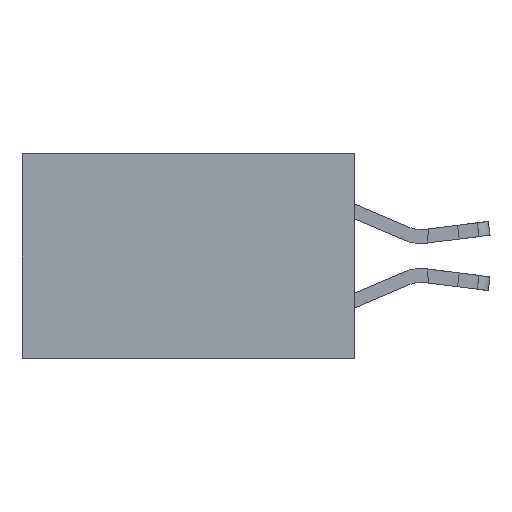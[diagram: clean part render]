
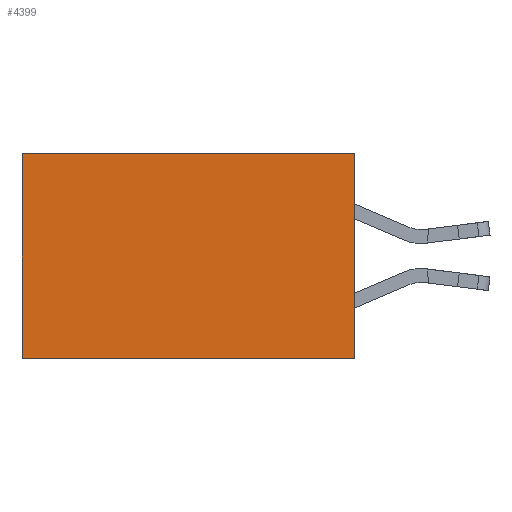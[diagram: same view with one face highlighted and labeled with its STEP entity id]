
A CAD part, left-side view. The second image highlights one B-rep face of the part: STEP entity #4399.
In plain terms, the highlighted planar face has unit normal (-1, 0, 0).
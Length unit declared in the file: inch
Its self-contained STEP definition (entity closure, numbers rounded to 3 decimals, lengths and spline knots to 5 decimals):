
#793 = VERTEX_POINT ( 'NONE', #21311 ) ;
#807 = LINE ( 'NONE', #1148, #21305 ) ;
#1148 = CARTESIAN_POINT ( 'NONE',  ( 0.2615, 0., 0. ) ) ;
#1713 = EDGE_LOOP ( 'NONE', ( #18513, #17192, #12336, #5022 ) ) ;
#2578 = PLANE ( 'NONE',  #19515 ) ;
#4399 = ADVANCED_FACE ( 'NONE', ( #13507 ), #2578, .F. ) ;
#4683 = VECTOR ( 'NONE', #21081, 39.37008 ) ;
#5022 = ORIENTED_EDGE ( 'NONE', *, *, #13475, .T. ) ;
#5232 = DIRECTION ( 'NONE',  ( 0., 1., 0. ) ) ;
#6463 = DIRECTION ( 'NONE',  ( 0., 0., -1. ) ) ;
#7161 = CARTESIAN_POINT ( 'NONE',  ( 0.2615, 0., -0.37 ) ) ;
#7286 = LINE ( 'NONE', #7161, #22339 ) ;
#7568 = CARTESIAN_POINT ( 'NONE',  ( 0.2615, 0., 0. ) ) ;
#7781 = VECTOR ( 'NONE', #6463, 39.37008 ) ;
#8053 = DIRECTION ( 'NONE',  ( 0., 0., -1. ) ) ;
#9041 = CARTESIAN_POINT ( 'NONE',  ( 0.2615, 0.6, 0. ) ) ;
#9795 = EDGE_CURVE ( 'NONE', #793, #12988, #7286, .T. ) ;
#10044 = DIRECTION ( 'NONE',  ( 0., 1., 0. ) ) ;
#12336 = ORIENTED_EDGE ( 'NONE', *, *, #17392, .F. ) ;
#12988 = VERTEX_POINT ( 'NONE', #17609 ) ;
#13475 = EDGE_CURVE ( 'NONE', #15215, #17031, #807, .T. ) ;
#13507 = FACE_OUTER_BOUND ( 'NONE', #1713, .T. ) ;
#15215 = VERTEX_POINT ( 'NONE', #7568 ) ;
#15832 = LINE ( 'NONE', #19357, #7781 ) ;
#17031 = VERTEX_POINT ( 'NONE', #9041 ) ;
#17192 = ORIENTED_EDGE ( 'NONE', *, *, #9795, .F. ) ;
#17329 = EDGE_CURVE ( 'NONE', #17031, #12988, #17434, .T. ) ;
#17392 = EDGE_CURVE ( 'NONE', #15215, #793, #15832, .T. ) ;
#17434 = LINE ( 'NONE', #19237, #4683 ) ;
#17609 = CARTESIAN_POINT ( 'NONE',  ( 0.2615, 0.6, -0.37 ) ) ;
#18513 = ORIENTED_EDGE ( 'NONE', *, *, #17329, .T. ) ;
#19116 = DIRECTION ( 'NONE',  ( 1., 0., 0. ) ) ;
#19237 = CARTESIAN_POINT ( 'NONE',  ( 0.2615, 0.6, -0.37 ) ) ;
#19357 = CARTESIAN_POINT ( 'NONE',  ( 0.2615, 0., -0.37 ) ) ;
#19515 = AXIS2_PLACEMENT_3D ( 'NONE', #21299, #19116, #8053 ) ;
#21081 = DIRECTION ( 'NONE',  ( 0., 0., -1. ) ) ;
#21299 = CARTESIAN_POINT ( 'NONE',  ( 0.2615, 0., -0.37 ) ) ;
#21305 = VECTOR ( 'NONE', #10044, 39.37008 ) ;
#21311 = CARTESIAN_POINT ( 'NONE',  ( 0.2615, 0., -0.37 ) ) ;
#22339 = VECTOR ( 'NONE', #5232, 39.37008 ) ;
